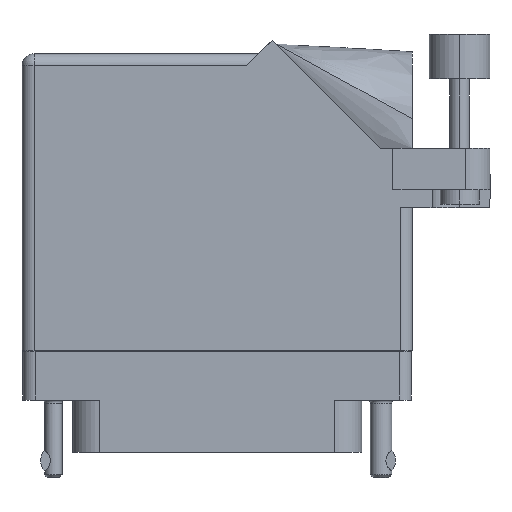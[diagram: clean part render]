
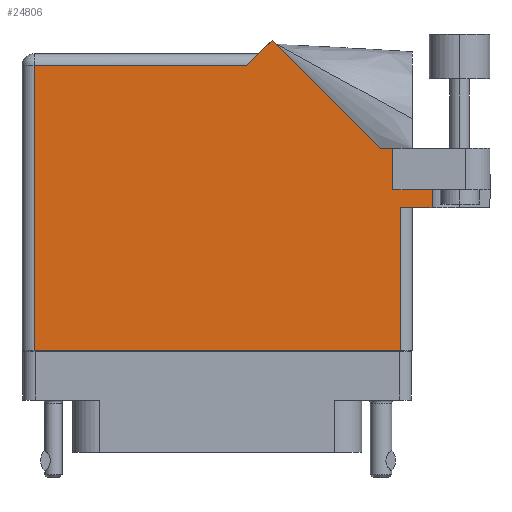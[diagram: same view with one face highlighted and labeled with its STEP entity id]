
A CAD part, front view. The second image highlights one B-rep face of the part: STEP entity #24806.
In plain terms, the highlighted face is planar.
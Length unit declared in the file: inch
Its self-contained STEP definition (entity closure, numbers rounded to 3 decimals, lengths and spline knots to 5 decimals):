
#120 = VERTEX_POINT ( 'NONE', #27905 ) ;
#338 = LINE ( 'NONE', #26217, #21900 ) ;
#475 = DIRECTION ( 'NONE',  ( 1., 0., 0. ) ) ;
#859 = CARTESIAN_POINT ( 'NONE',  ( 1.1065, 0.637, 0.455 ) ) ;
#1104 = CARTESIAN_POINT ( 'NONE',  ( -1.005, -0.1, 0.455 ) ) ;
#1754 = ORIENTED_EDGE ( 'NONE', *, *, #7963, .T. ) ;
#2256 = ORIENTED_EDGE ( 'NONE', *, *, #37310, .T. ) ;
#2368 = ORIENTED_EDGE ( 'NONE', *, *, #6404, .T. ) ;
#2949 = DIRECTION ( 'NONE',  ( 0., -1., 0. ) ) ;
#3637 = EDGE_CURVE ( 'NONE', #23902, #23125, #38607, .T. ) ;
#6295 = CARTESIAN_POINT ( 'NONE',  ( -0.943, -0.1, 0.455 ) ) ;
#6404 = EDGE_CURVE ( 'NONE', #28812, #20797, #32368, .T. ) ;
#6594 = LINE ( 'NONE', #49037, #8354 ) ;
#6703 = CARTESIAN_POINT ( 'NONE',  ( 0.28271, 1.50071, 0.455 ) ) ;
#7032 = VECTOR ( 'NONE', #39269, 39.37008 ) ;
#7587 = DIRECTION ( 'NONE',  ( -1., 0., 0. ) ) ;
#7692 = VECTOR ( 'NONE', #46356, 39.37008 ) ;
#7745 = VERTEX_POINT ( 'NONE', #15606 ) ;
#7963 = EDGE_CURVE ( 'NONE', #120, #34277, #26869, .T. ) ;
#8354 = VECTOR ( 'NONE', #30311, 39.37008 ) ;
#8451 = DIRECTION ( 'NONE',  ( -1., 0., 0. ) ) ;
#8614 = DIRECTION ( 'NONE',  ( 0., 0., -1. ) ) ;
#8861 = ORIENTED_EDGE ( 'NONE', *, *, #11243, .F. ) ;
#9108 = EDGE_CURVE ( 'NONE', #20797, #7745, #19022, .T. ) ;
#9304 = ORIENTED_EDGE ( 'NONE', *, *, #20483, .T. ) ;
#11243 = EDGE_CURVE ( 'NONE', #16840, #21496, #338, .T. ) ;
#11428 = DIRECTION ( 'NONE',  ( -0.707, -0.707, 0. ) ) ;
#12038 = LINE ( 'NONE', #6295, #40836 ) ;
#12291 = CARTESIAN_POINT ( 'NONE',  ( -1.005, 1.43, 0.455 ) ) ;
#13428 = ORIENTED_EDGE ( 'NONE', *, *, #14097, .T. ) ;
#14097 = EDGE_CURVE ( 'NONE', #23125, #28812, #12038, .T. ) ;
#14362 = CARTESIAN_POINT ( 'NONE',  ( -0.943, 1.368, 0.455 ) ) ;
#14462 = CARTESIAN_POINT ( 'NONE',  ( 0.905, 0.944, 0.455 ) ) ;
#14648 = CARTESIAN_POINT ( 'NONE',  ( 0.905, 0.731, 0.455 ) ) ;
#14891 = CARTESIAN_POINT ( 'NONE',  ( -1.005, 1.368, 0.455 ) ) ;
#15606 = CARTESIAN_POINT ( 'NONE',  ( 0.943, 0.637, 0.455 ) ) ;
#16840 = VERTEX_POINT ( 'NONE', #25756 ) ;
#17296 = AXIS2_PLACEMENT_3D ( 'NONE', #12291, #8614, #8451 ) ;
#17377 = VECTOR ( 'NONE', #28249, 39.37008 ) ;
#17463 = LINE ( 'NONE', #49625, #22258 ) ;
#18180 = LINE ( 'NONE', #19564, #39774 ) ;
#18773 = DIRECTION ( 'NONE',  ( -1., 0., 0. ) ) ;
#19022 = LINE ( 'NONE', #24347, #7032 ) ;
#19202 = EDGE_CURVE ( 'NONE', #7745, #21496, #18180, .T. ) ;
#19310 = CARTESIAN_POINT ( 'NONE',  ( 1.405, 0.944, 0.455 ) ) ;
#19564 = CARTESIAN_POINT ( 'NONE',  ( 1.005, 0.637, 0.455 ) ) ;
#20384 = ORIENTED_EDGE ( 'NONE', *, *, #19202, .T. ) ;
#20483 = EDGE_CURVE ( 'NONE', #34277, #23902, #17463, .T. ) ;
#20797 = VERTEX_POINT ( 'NONE', #38798 ) ;
#21256 = DIRECTION ( 'NONE',  ( 0., 1., 0. ) ) ;
#21496 = VERTEX_POINT ( 'NONE', #859 ) ;
#21696 = LINE ( 'NONE', #19310, #29482 ) ;
#21900 = VECTOR ( 'NONE', #40971, 39.37008 ) ;
#22258 = VECTOR ( 'NONE', #11428, 39.37008 ) ;
#22716 = VECTOR ( 'NONE', #21256, 39.37008 ) ;
#22813 = CARTESIAN_POINT ( 'NONE',  ( 0.83942, 0.944, 0.455 ) ) ;
#23125 = VERTEX_POINT ( 'NONE', #14362 ) ;
#23309 = LINE ( 'NONE', #14648, #22716 ) ;
#23902 = VERTEX_POINT ( 'NONE', #47369 ) ;
#24219 = VERTEX_POINT ( 'NONE', #14462 ) ;
#24347 = CARTESIAN_POINT ( 'NONE',  ( 0.943, 0.637, 0.455 ) ) ;
#24806 = ADVANCED_FACE ( 'NONE', ( #33453 ), #31742, .F. ) ;
#25756 = CARTESIAN_POINT ( 'NONE',  ( 1.1065, 0.731, 0.455 ) ) ;
#26217 = CARTESIAN_POINT ( 'NONE',  ( 1.1065, 1.06177, 0.455 ) ) ;
#26869 = LINE ( 'NONE', #22813, #7692 ) ;
#27905 = CARTESIAN_POINT ( 'NONE',  ( 0.83942, 0.944, 0.455 ) ) ;
#28249 = DIRECTION ( 'NONE',  ( 1., 0., 0. ) ) ;
#28609 = EDGE_LOOP ( 'NONE', ( #2368, #47851, #20384, #8861, #29296, #43156, #2256, #1754, #9304, #36805, #13428 ) ) ;
#28812 = VERTEX_POINT ( 'NONE', #46195 ) ;
#29296 = ORIENTED_EDGE ( 'NONE', *, *, #47429, .F. ) ;
#29482 = VECTOR ( 'NONE', #7587, 39.37008 ) ;
#30311 = DIRECTION ( 'NONE',  ( 1., 0., 0. ) ) ;
#31742 = PLANE ( 'NONE',  #17296 ) ;
#32368 = LINE ( 'NONE', #1104, #17377 ) ;
#32830 = EDGE_CURVE ( 'NONE', #36202, #24219, #23309, .T. ) ;
#33453 = FACE_OUTER_BOUND ( 'NONE', #28609, .T. ) ;
#34277 = VERTEX_POINT ( 'NONE', #6703 ) ;
#36202 = VERTEX_POINT ( 'NONE', #40095 ) ;
#36805 = ORIENTED_EDGE ( 'NONE', *, *, #3637, .T. ) ;
#37310 = EDGE_CURVE ( 'NONE', #24219, #120, #21696, .T. ) ;
#38607 = LINE ( 'NONE', #14891, #41009 ) ;
#38798 = CARTESIAN_POINT ( 'NONE',  ( 0.943, -0.1, 0.455 ) ) ;
#39269 = DIRECTION ( 'NONE',  ( 0., 1., 0. ) ) ;
#39774 = VECTOR ( 'NONE', #475, 39.37008 ) ;
#40095 = CARTESIAN_POINT ( 'NONE',  ( 0.905, 0.731, 0.455 ) ) ;
#40836 = VECTOR ( 'NONE', #2949, 39.37008 ) ;
#40971 = DIRECTION ( 'NONE',  ( 0., -1., 0. ) ) ;
#41009 = VECTOR ( 'NONE', #18773, 39.37008 ) ;
#43156 = ORIENTED_EDGE ( 'NONE', *, *, #32830, .T. ) ;
#46195 = CARTESIAN_POINT ( 'NONE',  ( -0.943, -0.1, 0.455 ) ) ;
#46356 = DIRECTION ( 'NONE',  ( -0.707, 0.707, 0. ) ) ;
#47369 = CARTESIAN_POINT ( 'NONE',  ( 0.15, 1.368, 0.455 ) ) ;
#47429 = EDGE_CURVE ( 'NONE', #36202, #16840, #6594, .T. ) ;
#47851 = ORIENTED_EDGE ( 'NONE', *, *, #9108, .T. ) ;
#49037 = CARTESIAN_POINT ( 'NONE',  ( 0.905, 0.731, 0.455 ) ) ;
#49625 = CARTESIAN_POINT ( 'NONE',  ( 0.212, 1.43, 0.455 ) ) ;
